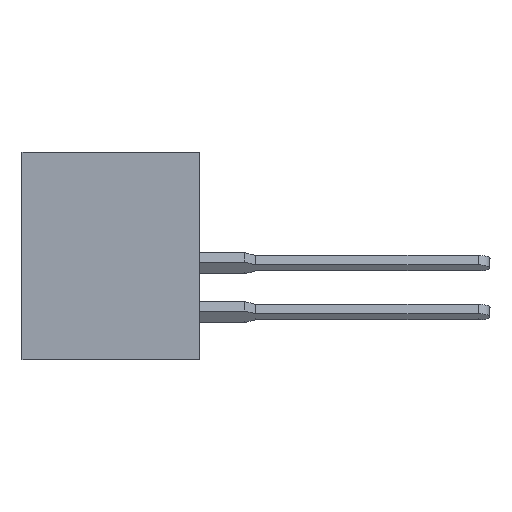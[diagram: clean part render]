
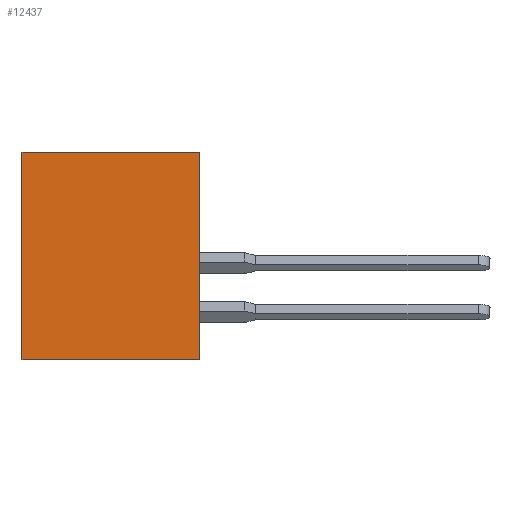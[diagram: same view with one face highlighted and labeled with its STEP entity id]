
A CAD part, left-side view. The second image highlights one B-rep face of the part: STEP entity #12437.
In plain terms, the highlighted planar face has unit normal (-1, 0, 0).
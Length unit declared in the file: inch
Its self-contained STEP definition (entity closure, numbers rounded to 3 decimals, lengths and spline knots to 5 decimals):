
#650 = ORIENTED_EDGE ( 'NONE', *, *, #19390, .T. ) ;
#1137 = CARTESIAN_POINT ( 'NONE',  ( 0., 0., 0. ) ) ;
#2012 = EDGE_LOOP ( 'NONE', ( #19562, #9297, #12998, #650 ) ) ;
#3855 = FACE_OUTER_BOUND ( 'NONE', #2012, .T. ) ;
#5331 = VECTOR ( 'NONE', #12684, 39.37008 ) ;
#5700 = PLANE ( 'NONE',  #11028 ) ;
#5781 = DIRECTION ( 'NONE',  ( 1., 0., 0. ) ) ;
#5902 = VECTOR ( 'NONE', #8851, 39.37008 ) ;
#5979 = VERTEX_POINT ( 'NONE', #20936 ) ;
#6459 = LINE ( 'NONE', #7327, #5331 ) ;
#6619 = LINE ( 'NONE', #9240, #15193 ) ;
#6924 = CARTESIAN_POINT ( 'NONE',  ( 0., 0.453, 0. ) ) ;
#7327 = CARTESIAN_POINT ( 'NONE',  ( 0., 0.453, 0. ) ) ;
#8236 = CARTESIAN_POINT ( 'NONE',  ( 0., 0.453, 0. ) ) ;
#8851 = DIRECTION ( 'NONE',  ( 0., -1., 0. ) ) ;
#9240 = CARTESIAN_POINT ( 'NONE',  ( 0., 0.453, -0.531 ) ) ;
#9297 = ORIENTED_EDGE ( 'NONE', *, *, #22917, .F. ) ;
#10750 = VERTEX_POINT ( 'NONE', #12543 ) ;
#11028 = AXIS2_PLACEMENT_3D ( 'NONE', #16393, #5781, #21384 ) ;
#12437 = ADVANCED_FACE ( 'NONE', ( #3855 ), #5700, .F. ) ;
#12543 = CARTESIAN_POINT ( 'NONE',  ( 0., 0.453, -0.531 ) ) ;
#12684 = DIRECTION ( 'NONE',  ( 0., 0., 1. ) ) ;
#12819 = VECTOR ( 'NONE', #20641, 39.37008 ) ;
#12998 = ORIENTED_EDGE ( 'NONE', *, *, #16285, .F. ) ;
#15193 = VECTOR ( 'NONE', #16123, 39.37008 ) ;
#15327 = LINE ( 'NONE', #6924, #5902 ) ;
#15386 = VERTEX_POINT ( 'NONE', #20661 ) ;
#16123 = DIRECTION ( 'NONE',  ( 0., -1., 0. ) ) ;
#16285 = EDGE_CURVE ( 'NONE', #10750, #16364, #6459, .T. ) ;
#16364 = VERTEX_POINT ( 'NONE', #8236 ) ;
#16393 = CARTESIAN_POINT ( 'NONE',  ( 0., 0.453, 0. ) ) ;
#16529 = EDGE_CURVE ( 'NONE', #15386, #5979, #17809, .T. ) ;
#17809 = LINE ( 'NONE', #1137, #12819 ) ;
#19390 = EDGE_CURVE ( 'NONE', #10750, #15386, #6619, .T. ) ;
#19562 = ORIENTED_EDGE ( 'NONE', *, *, #16529, .T. ) ;
#20641 = DIRECTION ( 'NONE',  ( 0., 0., 1. ) ) ;
#20661 = CARTESIAN_POINT ( 'NONE',  ( 0., 0., -0.531 ) ) ;
#20936 = CARTESIAN_POINT ( 'NONE',  ( 0., 0., 0. ) ) ;
#21384 = DIRECTION ( 'NONE',  ( 0., 0., -1. ) ) ;
#22917 = EDGE_CURVE ( 'NONE', #16364, #5979, #15327, .T. ) ;
